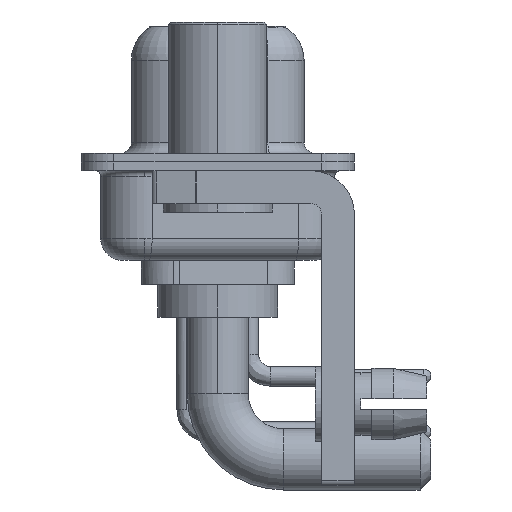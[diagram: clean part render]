
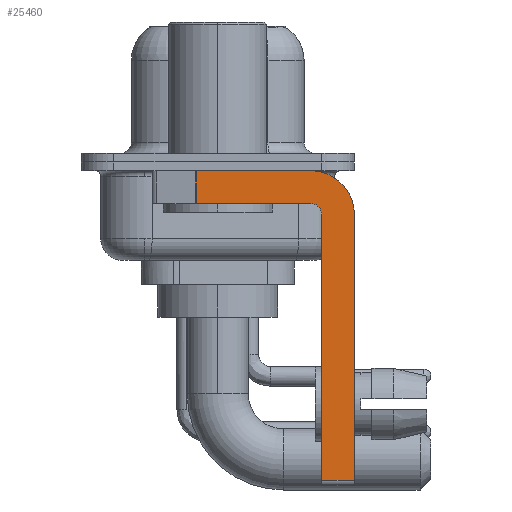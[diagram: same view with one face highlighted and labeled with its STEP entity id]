
A CAD part, left-side view. The second image highlights one B-rep face of the part: STEP entity #25460.
In plain terms, the highlighted planar face has unit normal (-1, 0, 0).
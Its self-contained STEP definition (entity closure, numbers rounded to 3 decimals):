
#215 = VERTEX_POINT ( 'NONE', #2930 ) ;
#433 = VERTEX_POINT ( 'NONE', #23850 ) ;
#446 = FACE_OUTER_BOUND ( 'NONE', #7522, .T. ) ;
#563 = ORIENTED_EDGE ( 'NONE', *, *, #13417, .F. ) ;
#716 = DIRECTION ( 'NONE',  ( 0., 0., -1. ) ) ;
#930 = CARTESIAN_POINT ( 'NONE',  ( -2.9, -4.25, -0.4 ) ) ;
#981 = AXIS2_PLACEMENT_3D ( 'NONE', #10525, #18443, #716 ) ;
#1299 = VECTOR ( 'NONE', #8163, 1000. ) ;
#1587 = DIRECTION ( 'NONE',  ( 0., 0., 1. ) ) ;
#2067 = CARTESIAN_POINT ( 'NONE',  ( -2.9, -4.25, -1.9 ) ) ;
#2308 = EDGE_CURVE ( 'NONE', #8145, #2371, #13766, .T. ) ;
#2371 = VERTEX_POINT ( 'NONE', #16050 ) ;
#2405 = ORIENTED_EDGE ( 'NONE', *, *, #14759, .F. ) ;
#2701 = LINE ( 'NONE', #2820, #24478 ) ;
#2780 = VERTEX_POINT ( 'NONE', #16595 ) ;
#2820 = CARTESIAN_POINT ( 'NONE',  ( -2.9, -6.25, -2.4 ) ) ;
#2930 = CARTESIAN_POINT ( 'NONE',  ( -2.9, -6.25, -14.55 ) ) ;
#6408 = DIRECTION ( 'NONE',  ( 1., 0., 0. ) ) ;
#6561 = CARTESIAN_POINT ( 'NONE',  ( -2.9, 3., -0.4 ) ) ;
#6582 = DIRECTION ( 'NONE',  ( 0., 0., -1. ) ) ;
#6986 = VECTOR ( 'NONE', #18258, 1000. ) ;
#7450 = VERTEX_POINT ( 'NONE', #7713 ) ;
#7510 = DIRECTION ( 'NONE',  ( 0., 1., 0. ) ) ;
#7522 = EDGE_LOOP ( 'NONE', ( #563, #13457, #22662, #8218, #2405, #15456, #12540, #13228 ) ) ;
#7713 = CARTESIAN_POINT ( 'NONE',  ( -2.9, -4.75, -2.4 ) ) ;
#7779 = CARTESIAN_POINT ( 'NONE',  ( -2.9, -4.25, -1.9 ) ) ;
#8145 = VERTEX_POINT ( 'NONE', #930 ) ;
#8163 = DIRECTION ( 'NONE',  ( 0., 0., 1. ) ) ;
#8218 = ORIENTED_EDGE ( 'NONE', *, *, #18078, .F. ) ;
#8338 = CARTESIAN_POINT ( 'NONE',  ( -2.9, -4.25, -2.4 ) ) ;
#9486 = VECTOR ( 'NONE', #20150, 1000. ) ;
#10030 = EDGE_CURVE ( 'NONE', #2780, #215, #20829, .T. ) ;
#10083 = CARTESIAN_POINT ( 'NONE',  ( -2.9, -4.75, -14.8 ) ) ;
#10258 = PLANE ( 'NONE',  #17089 ) ;
#10525 = CARTESIAN_POINT ( 'NONE',  ( -2.9, -4.25, -2.4 ) ) ;
#10750 = VECTOR ( 'NONE', #7510, 1000. ) ;
#11036 = VERTEX_POINT ( 'NONE', #7779 ) ;
#11245 = EDGE_CURVE ( 'NONE', #433, #17392, #15918, .T. ) ;
#11765 = LINE ( 'NONE', #10083, #1299 ) ;
#12540 = ORIENTED_EDGE ( 'NONE', *, *, #16696, .F. ) ;
#12887 = EDGE_CURVE ( 'NONE', #11036, #17392, #15391, .T. ) ;
#13055 = DIRECTION ( 'NONE',  ( 0., -1., 0. ) ) ;
#13228 = ORIENTED_EDGE ( 'NONE', *, *, #2308, .F. ) ;
#13345 = DIRECTION ( 'NONE',  ( -1., 0., 0. ) ) ;
#13417 = EDGE_CURVE ( 'NONE', #433, #8145, #16385, .T. ) ;
#13457 = ORIENTED_EDGE ( 'NONE', *, *, #11245, .T. ) ;
#13766 = CIRCLE ( 'NONE', #981, 2. ) ;
#14759 = EDGE_CURVE ( 'NONE', #2780, #7450, #11765, .T. ) ;
#15187 = VECTOR ( 'NONE', #13055, 1000. ) ;
#15391 = LINE ( 'NONE', #2067, #10750 ) ;
#15456 = ORIENTED_EDGE ( 'NONE', *, *, #10030, .T. ) ;
#15878 = CIRCLE ( 'NONE', #19210, 0.5 ) ;
#15918 = LINE ( 'NONE', #23811, #6986 ) ;
#16050 = CARTESIAN_POINT ( 'NONE',  ( -2.9, -6.25, -2.4 ) ) ;
#16385 = LINE ( 'NONE', #6561, #9486 ) ;
#16595 = CARTESIAN_POINT ( 'NONE',  ( -2.9, -4.75, -14.55 ) ) ;
#16696 = EDGE_CURVE ( 'NONE', #2371, #215, #2701, .T. ) ;
#17089 = AXIS2_PLACEMENT_3D ( 'NONE', #8338, #6408, #18167 ) ;
#17392 = VERTEX_POINT ( 'NONE', #23086 ) ;
#18078 = EDGE_CURVE ( 'NONE', #7450, #11036, #15878, .T. ) ;
#18167 = DIRECTION ( 'NONE',  ( 0., 0., -1. ) ) ;
#18258 = DIRECTION ( 'NONE',  ( 0., 0., -1. ) ) ;
#18443 = DIRECTION ( 'NONE',  ( 1., 0., 0. ) ) ;
#19210 = AXIS2_PLACEMENT_3D ( 'NONE', #23185, #13345, #1587 ) ;
#20150 = DIRECTION ( 'NONE',  ( 0., -1., 0. ) ) ;
#20829 = LINE ( 'NONE', #24963, #15187 ) ;
#22662 = ORIENTED_EDGE ( 'NONE', *, *, #12887, .F. ) ;
#23086 = CARTESIAN_POINT ( 'NONE',  ( -2.9, 0.978, -1.9 ) ) ;
#23185 = CARTESIAN_POINT ( 'NONE',  ( -2.9, -4.25, -2.4 ) ) ;
#23811 = CARTESIAN_POINT ( 'NONE',  ( -2.9, 0.978, -1.9 ) ) ;
#23850 = CARTESIAN_POINT ( 'NONE',  ( -2.9, 0.978, -0.4 ) ) ;
#24478 = VECTOR ( 'NONE', #6582, 1000. ) ;
#24963 = CARTESIAN_POINT ( 'NONE',  ( -2.9, -4.25, -14.55 ) ) ;
#25460 = ADVANCED_FACE ( 'NONE', ( #446 ), #10258, .F. ) ;
